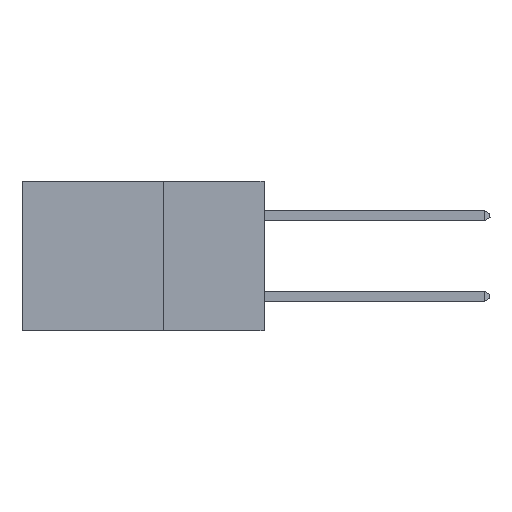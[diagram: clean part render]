
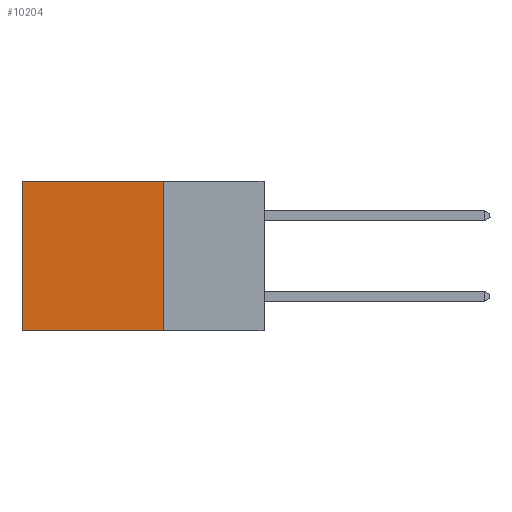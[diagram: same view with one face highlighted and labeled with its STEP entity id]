
A CAD part, left-side view. The second image highlights one B-rep face of the part: STEP entity #10204.
In plain terms, the highlighted planar face has unit normal (-1, 0, 0).
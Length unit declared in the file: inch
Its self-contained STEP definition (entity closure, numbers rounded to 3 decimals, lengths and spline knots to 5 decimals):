
#917 = CARTESIAN_POINT ( 'NONE',  ( 0.298, 0.25, -0.37 ) ) ;
#1126 = CARTESIAN_POINT ( 'NONE',  ( 0.298, 0.6, 0. ) ) ;
#1596 = CARTESIAN_POINT ( 'NONE',  ( 0.298, 0.6, -0.37 ) ) ;
#2043 = DIRECTION ( 'NONE',  ( 0., 0., -1. ) ) ;
#3599 = EDGE_LOOP ( 'NONE', ( #23495, #5272, #8343, #17765 ) ) ;
#3834 = LINE ( 'NONE', #917, #29269 ) ;
#5272 = ORIENTED_EDGE ( 'NONE', *, *, #11592, .F. ) ;
#5664 = DIRECTION ( 'NONE',  ( 0., 1., 0. ) ) ;
#6401 = EDGE_CURVE ( 'NONE', #22360, #8996, #14991, .T. ) ;
#7574 = EDGE_CURVE ( 'NONE', #22360, #26799, #22019, .T. ) ;
#8343 = ORIENTED_EDGE ( 'NONE', *, *, #6401, .F. ) ;
#8673 = EDGE_CURVE ( 'NONE', #26799, #9821, #15255, .T. ) ;
#8992 = VECTOR ( 'NONE', #2043, 39.37008 ) ;
#8996 = VERTEX_POINT ( 'NONE', #20060 ) ;
#9172 = CARTESIAN_POINT ( 'NONE',  ( 0.298, 0.25, 0. ) ) ;
#9539 = DIRECTION ( 'NONE',  ( 0., 1., 0. ) ) ;
#9800 = CARTESIAN_POINT ( 'NONE',  ( 0.298, 0.6, 0. ) ) ;
#9821 = VERTEX_POINT ( 'NONE', #1596 ) ;
#10204 = ADVANCED_FACE ( 'NONE', ( #13379 ), #25157, .F. ) ;
#11592 = EDGE_CURVE ( 'NONE', #8996, #9821, #3834, .T. ) ;
#11615 = DIRECTION ( 'NONE',  ( 0., 0., -1. ) ) ;
#11717 = DIRECTION ( 'NONE',  ( 1., 0., 0. ) ) ;
#11826 = CARTESIAN_POINT ( 'NONE',  ( 0.298, 0.25, 0. ) ) ;
#11978 = DIRECTION ( 'NONE',  ( 0., 0., -1. ) ) ;
#13379 = FACE_OUTER_BOUND ( 'NONE', #3599, .T. ) ;
#14991 = LINE ( 'NONE', #9172, #8992 ) ;
#15255 = LINE ( 'NONE', #9800, #23401 ) ;
#17765 = ORIENTED_EDGE ( 'NONE', *, *, #7574, .T. ) ;
#18420 = CARTESIAN_POINT ( 'NONE',  ( 0.298, 0.25, 0. ) ) ;
#18465 = CARTESIAN_POINT ( 'NONE',  ( 0.298, 0.25, 0. ) ) ;
#18842 = VECTOR ( 'NONE', #9539, 39.37008 ) ;
#20060 = CARTESIAN_POINT ( 'NONE',  ( 0.298, 0.25, -0.37 ) ) ;
#21435 = AXIS2_PLACEMENT_3D ( 'NONE', #18465, #11717, #11615 ) ;
#22019 = LINE ( 'NONE', #11826, #18842 ) ;
#22360 = VERTEX_POINT ( 'NONE', #18420 ) ;
#23401 = VECTOR ( 'NONE', #11978, 39.37008 ) ;
#23495 = ORIENTED_EDGE ( 'NONE', *, *, #8673, .T. ) ;
#25157 = PLANE ( 'NONE',  #21435 ) ;
#26799 = VERTEX_POINT ( 'NONE', #1126 ) ;
#29269 = VECTOR ( 'NONE', #5664, 39.37008 ) ;
